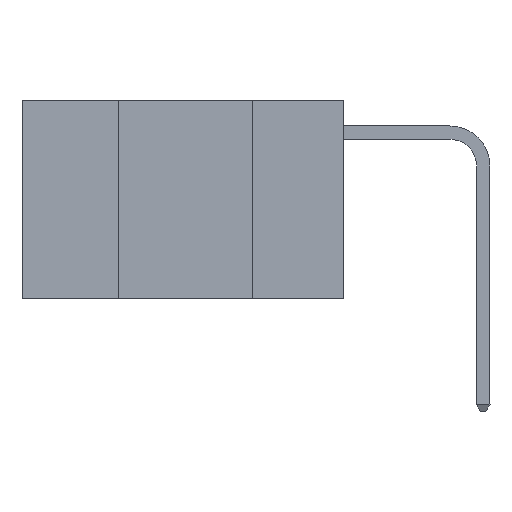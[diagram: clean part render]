
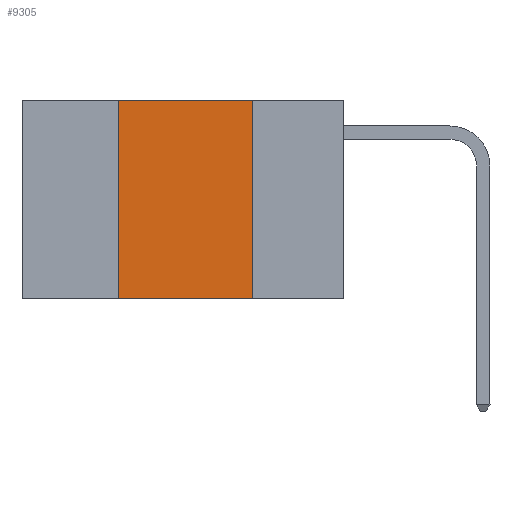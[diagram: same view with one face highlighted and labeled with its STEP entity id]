
A CAD part, left-side view. The second image highlights one B-rep face of the part: STEP entity #9305.
In plain terms, the highlighted planar face has unit normal (-1, 0, 0).
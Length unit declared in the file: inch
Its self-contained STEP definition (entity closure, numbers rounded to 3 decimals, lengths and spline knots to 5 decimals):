
#188 = DIRECTION ( 'NONE',  ( 0., 0., -1. ) ) ;
#616 = VERTEX_POINT ( 'NONE', #7085 ) ;
#1323 = VECTOR ( 'NONE', #1637, 39.37008 ) ;
#1564 = DIRECTION ( 'NONE',  ( 0., -1., 0. ) ) ;
#1637 = DIRECTION ( 'NONE',  ( 0., 0., 1. ) ) ;
#2758 = CARTESIAN_POINT ( 'NONE',  ( 0., 0.6, 0. ) ) ;
#2838 = CARTESIAN_POINT ( 'NONE',  ( 0., 0.42, 0. ) ) ;
#3034 = VERTEX_POINT ( 'NONE', #9173 ) ;
#3973 = CARTESIAN_POINT ( 'NONE',  ( 0., 0.17, 0. ) ) ;
#4598 = VECTOR ( 'NONE', #1564, 39.37008 ) ;
#4746 = EDGE_CURVE ( 'NONE', #3034, #616, #10369, .T. ) ;
#5537 = DIRECTION ( 'NONE',  ( 0., -1., 0. ) ) ;
#5922 = PLANE ( 'NONE',  #11567 ) ;
#6527 = ORIENTED_EDGE ( 'NONE', *, *, #7335, .F. ) ;
#7010 = ORIENTED_EDGE ( 'NONE', *, *, #7951, .F. ) ;
#7040 = CARTESIAN_POINT ( 'NONE',  ( 0., 0.17, 0. ) ) ;
#7085 = CARTESIAN_POINT ( 'NONE',  ( 0., 0.17, -0.37 ) ) ;
#7105 = DIRECTION ( 'NONE',  ( 1., 0., 0. ) ) ;
#7306 = EDGE_CURVE ( 'NONE', #3034, #8857, #10320, .T. ) ;
#7335 = EDGE_CURVE ( 'NONE', #13299, #616, #13376, .T. ) ;
#7463 = DIRECTION ( 'NONE',  ( 0., 0., -1. ) ) ;
#7487 = VECTOR ( 'NONE', #7463, 39.37008 ) ;
#7645 = LINE ( 'NONE', #2758, #4598 ) ;
#7951 = EDGE_CURVE ( 'NONE', #8857, #13299, #7645, .T. ) ;
#8210 = EDGE_LOOP ( 'NONE', ( #6527, #7010, #10619, #12362 ) ) ;
#8262 = VECTOR ( 'NONE', #5537, 39.37008 ) ;
#8857 = VERTEX_POINT ( 'NONE', #2838 ) ;
#9143 = FACE_OUTER_BOUND ( 'NONE', #8210, .T. ) ;
#9173 = CARTESIAN_POINT ( 'NONE',  ( 0., 0.42, -0.37 ) ) ;
#9305 = ADVANCED_FACE ( 'NONE', ( #9143 ), #5922, .F. ) ;
#10320 = LINE ( 'NONE', #13674, #1323 ) ;
#10369 = LINE ( 'NONE', #13042, #8262 ) ;
#10619 = ORIENTED_EDGE ( 'NONE', *, *, #7306, .F. ) ;
#11567 = AXIS2_PLACEMENT_3D ( 'NONE', #12388, #7105, #188 ) ;
#12362 = ORIENTED_EDGE ( 'NONE', *, *, #4746, .T. ) ;
#12388 = CARTESIAN_POINT ( 'NONE',  ( 0., 0.6, 0. ) ) ;
#13042 = CARTESIAN_POINT ( 'NONE',  ( 0., 0.6, -0.37 ) ) ;
#13299 = VERTEX_POINT ( 'NONE', #7040 ) ;
#13376 = LINE ( 'NONE', #3973, #7487 ) ;
#13674 = CARTESIAN_POINT ( 'NONE',  ( 0., 0.42, 0. ) ) ;
